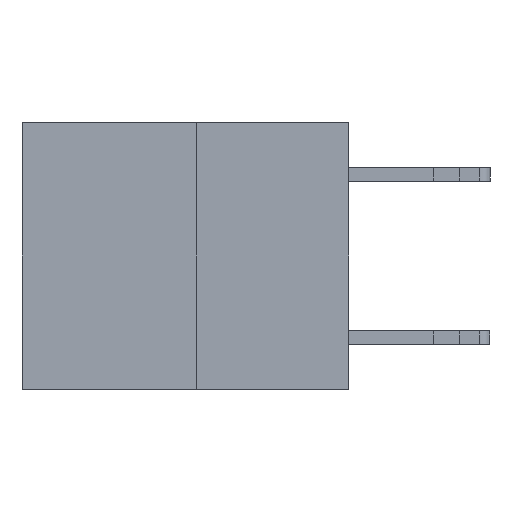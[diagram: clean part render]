
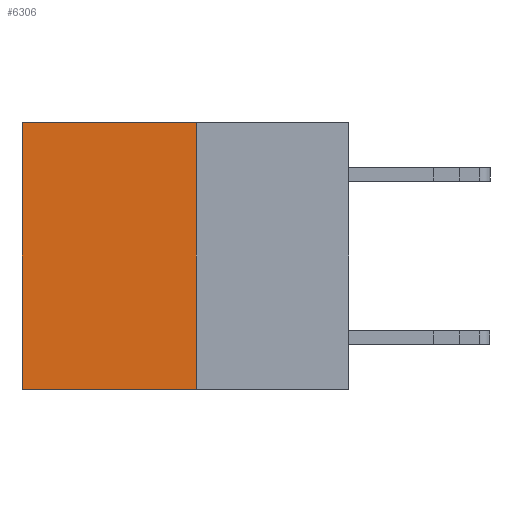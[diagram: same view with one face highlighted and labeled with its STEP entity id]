
A CAD part, left-side view. The second image highlights one B-rep face of the part: STEP entity #6306.
In plain terms, the highlighted planar face has unit normal (-1, 0, 0).
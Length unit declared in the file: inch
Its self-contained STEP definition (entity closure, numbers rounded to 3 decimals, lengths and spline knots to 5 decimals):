
#35 = DIRECTION ( 'NONE',  ( 0., 0., -1. ) ) ;
#178 = CARTESIAN_POINT ( 'NONE',  ( 0.3165, 0.28, 0. ) ) ;
#514 = AXIS2_PLACEMENT_3D ( 'NONE', #3572, #8336, #14450 ) ;
#848 = VERTEX_POINT ( 'NONE', #178 ) ;
#1257 = VECTOR ( 'NONE', #7718, 39.37008 ) ;
#1321 = ORIENTED_EDGE ( 'NONE', *, *, #9831, .T. ) ;
#1489 = VECTOR ( 'NONE', #9133, 39.37008 ) ;
#2242 = DIRECTION ( 'NONE',  ( 0., 1., 0. ) ) ;
#2288 = EDGE_LOOP ( 'NONE', ( #8994, #3039, #5689, #1321 ) ) ;
#2323 = EDGE_CURVE ( 'NONE', #848, #2607, #15008, .T. ) ;
#2607 = VERTEX_POINT ( 'NONE', #2946 ) ;
#2871 = FACE_OUTER_BOUND ( 'NONE', #2288, .T. ) ;
#2946 = CARTESIAN_POINT ( 'NONE',  ( 0.3165, 0.28, -0.49 ) ) ;
#3039 = ORIENTED_EDGE ( 'NONE', *, *, #11958, .F. ) ;
#3517 = CARTESIAN_POINT ( 'NONE',  ( 0.3165, 0.28, -0.49 ) ) ;
#3566 = CARTESIAN_POINT ( 'NONE',  ( 0.3165, 0.28, -0.49 ) ) ;
#3572 = CARTESIAN_POINT ( 'NONE',  ( 0.3165, 0.28, -0.49 ) ) ;
#3874 = EDGE_CURVE ( 'NONE', #11736, #7215, #5771, .T. ) ;
#4412 = CARTESIAN_POINT ( 'NONE',  ( 0.3165, 0.6, 0. ) ) ;
#4735 = LINE ( 'NONE', #11915, #10582 ) ;
#4854 = PLANE ( 'NONE',  #514 ) ;
#5689 = ORIENTED_EDGE ( 'NONE', *, *, #2323, .F. ) ;
#5771 = LINE ( 'NONE', #15002, #1257 ) ;
#6306 = ADVANCED_FACE ( 'NONE', ( #2871 ), #4854, .F. ) ;
#6547 = CARTESIAN_POINT ( 'NONE',  ( 0.3165, 0.6, -0.49 ) ) ;
#7215 = VERTEX_POINT ( 'NONE', #6547 ) ;
#7718 = DIRECTION ( 'NONE',  ( 0., 0., -1. ) ) ;
#8336 = DIRECTION ( 'NONE',  ( 1., 0., 0. ) ) ;
#8994 = ORIENTED_EDGE ( 'NONE', *, *, #3874, .T. ) ;
#9133 = DIRECTION ( 'NONE',  ( 0., 1., 0. ) ) ;
#9831 = EDGE_CURVE ( 'NONE', #848, #11736, #4735, .T. ) ;
#10582 = VECTOR ( 'NONE', #2242, 39.37008 ) ;
#11736 = VERTEX_POINT ( 'NONE', #4412 ) ;
#11915 = CARTESIAN_POINT ( 'NONE',  ( 0.3165, 0.28, 0. ) ) ;
#11958 = EDGE_CURVE ( 'NONE', #2607, #7215, #14171, .T. ) ;
#14171 = LINE ( 'NONE', #3566, #1489 ) ;
#14450 = DIRECTION ( 'NONE',  ( 0., 0., -1. ) ) ;
#14825 = VECTOR ( 'NONE', #35, 39.37008 ) ;
#15002 = CARTESIAN_POINT ( 'NONE',  ( 0.3165, 0.6, -0.49 ) ) ;
#15008 = LINE ( 'NONE', #3517, #14825 ) ;
